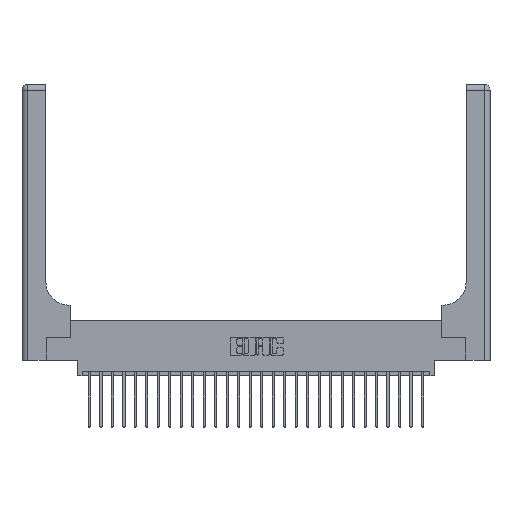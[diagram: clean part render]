
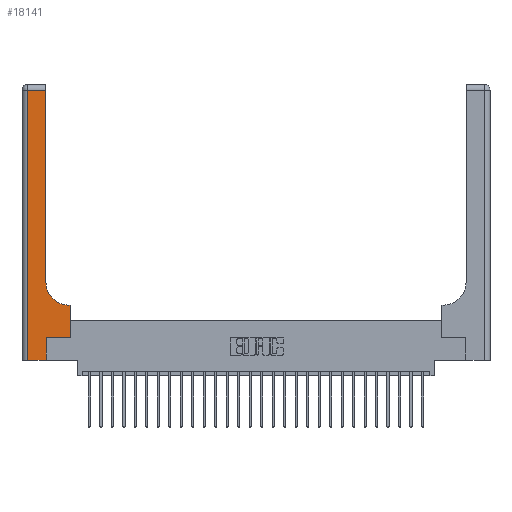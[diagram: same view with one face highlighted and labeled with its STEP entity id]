
A CAD part, top view. The second image highlights one B-rep face of the part: STEP entity #18141.
In plain terms, the highlighted planar face has unit normal (0, 0, 1).
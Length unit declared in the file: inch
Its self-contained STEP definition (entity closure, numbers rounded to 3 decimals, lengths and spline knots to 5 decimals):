
#2 = DIRECTION ( 'NONE',  ( 1., 0., 0. ) ) ;
#384 = DIRECTION ( 'NONE',  ( 0., 1., 0. ) ) ;
#414 = EDGE_CURVE ( 'NONE', #9148, #3747, #14140, .T. ) ;
#437 = CARTESIAN_POINT ( 'NONE',  ( 0.06, 3., 0.37 ) ) ;
#682 = CARTESIAN_POINT ( 'NONE',  ( 0.06, 0., 0.37 ) ) ;
#783 = CARTESIAN_POINT ( 'NONE',  ( 0.528, 0.6, 0.37 ) ) ;
#811 = DIRECTION ( 'NONE',  ( 1., 0., 0. ) ) ;
#1477 = LINE ( 'NONE', #24957, #22028 ) ;
#1727 = LINE ( 'NONE', #9113, #22916 ) ;
#2318 = DIRECTION ( 'NONE',  ( 1., 0., 0. ) ) ;
#2711 = VERTEX_POINT ( 'NONE', #22517 ) ;
#2744 = LINE ( 'NONE', #437, #19110 ) ;
#2953 = VERTEX_POINT ( 'NONE', #783 ) ;
#3747 = VERTEX_POINT ( 'NONE', #23976 ) ;
#4398 = CIRCLE ( 'NONE', #25524, 0.25 ) ;
#4482 = VECTOR ( 'NONE', #2318, 39.37008 ) ;
#4495 = LINE ( 'NONE', #6104, #14080 ) ;
#4912 = CARTESIAN_POINT ( 'NONE',  ( 0., 2.94, 0.37 ) ) ;
#4923 = FACE_OUTER_BOUND ( 'NONE', #15875, .T. ) ;
#5685 = VECTOR ( 'NONE', #19281, 39.37008 ) ;
#6093 = CARTESIAN_POINT ( 'NONE',  ( 0.51, 0.6, 0.37 ) ) ;
#6104 = CARTESIAN_POINT ( 'NONE',  ( 0.265, 0.25, 0.37 ) ) ;
#6271 = EDGE_CURVE ( 'NONE', #2711, #12326, #21415, .T. ) ;
#6777 = EDGE_CURVE ( 'NONE', #13794, #2711, #1477, .T. ) ;
#6854 = PLANE ( 'NONE',  #11545 ) ;
#7512 = ORIENTED_EDGE ( 'NONE', *, *, #14644, .T. ) ;
#7548 = CARTESIAN_POINT ( 'NONE',  ( 0.265, 0., 0.37 ) ) ;
#7654 = EDGE_CURVE ( 'NONE', #12326, #25879, #2744, .T. ) ;
#8391 = CARTESIAN_POINT ( 'NONE',  ( 0., 0., 0.37 ) ) ;
#8918 = DIRECTION ( 'NONE',  ( 0., 0., -1. ) ) ;
#9113 = CARTESIAN_POINT ( 'NONE',  ( 0.528, 0.25, 0.37 ) ) ;
#9148 = VERTEX_POINT ( 'NONE', #7548 ) ;
#10412 = EDGE_CURVE ( 'NONE', #22417, #13794, #4398, .T. ) ;
#10836 = ORIENTED_EDGE ( 'NONE', *, *, #17801, .T. ) ;
#11217 = DIRECTION ( 'NONE',  ( -1., 0., 0. ) ) ;
#11545 = AXIS2_PLACEMENT_3D ( 'NONE', #12942, #8918, #23276 ) ;
#11907 = CARTESIAN_POINT ( 'NONE',  ( 0.26, 0.85, 0.37 ) ) ;
#12326 = VERTEX_POINT ( 'NONE', #23500 ) ;
#12942 = CARTESIAN_POINT ( 'NONE',  ( 0., 3., 0.37 ) ) ;
#13046 = ORIENTED_EDGE ( 'NONE', *, *, #20359, .T. ) ;
#13093 = DIRECTION ( 'NONE',  ( 0., 1., 0. ) ) ;
#13095 = DIRECTION ( 'NONE',  ( 0., 0., -1. ) ) ;
#13794 = VERTEX_POINT ( 'NONE', #11907 ) ;
#14080 = VECTOR ( 'NONE', #2, 39.37008 ) ;
#14140 = LINE ( 'NONE', #21115, #19012 ) ;
#14644 = EDGE_CURVE ( 'NONE', #25879, #9148, #20851, .T. ) ;
#15049 = VECTOR ( 'NONE', #11217, 39.37008 ) ;
#15875 = EDGE_LOOP ( 'NONE', ( #20705, #19772, #24175, #7512, #19114, #13046, #10836, #22332, #19027 ) ) ;
#17546 = VERTEX_POINT ( 'NONE', #24544 ) ;
#17801 = EDGE_CURVE ( 'NONE', #17546, #2953, #1727, .T. ) ;
#18141 = ADVANCED_FACE ( 'NONE', ( #4923 ), #6854, .F. ) ;
#19012 = VECTOR ( 'NONE', #13093, 39.37008 ) ;
#19027 = ORIENTED_EDGE ( 'NONE', *, *, #10412, .T. ) ;
#19110 = VECTOR ( 'NONE', #20998, 39.37008 ) ;
#19114 = ORIENTED_EDGE ( 'NONE', *, *, #414, .T. ) ;
#19281 = DIRECTION ( 'NONE',  ( -1., 0., 0. ) ) ;
#19772 = ORIENTED_EDGE ( 'NONE', *, *, #6271, .T. ) ;
#20359 = EDGE_CURVE ( 'NONE', #3747, #17546, #4495, .T. ) ;
#20564 = LINE ( 'NONE', #21456, #15049 ) ;
#20705 = ORIENTED_EDGE ( 'NONE', *, *, #6777, .T. ) ;
#20851 = LINE ( 'NONE', #8391, #4482 ) ;
#20998 = DIRECTION ( 'NONE',  ( 0., -1., 0. ) ) ;
#21115 = CARTESIAN_POINT ( 'NONE',  ( 0.265, 0., 0.37 ) ) ;
#21415 = LINE ( 'NONE', #4912, #5685 ) ;
#21456 = CARTESIAN_POINT ( 'NONE',  ( 0.26, 0.6, 0.37 ) ) ;
#22028 = VECTOR ( 'NONE', #384, 39.37008 ) ;
#22332 = ORIENTED_EDGE ( 'NONE', *, *, #25313, .T. ) ;
#22417 = VERTEX_POINT ( 'NONE', #6093 ) ;
#22517 = CARTESIAN_POINT ( 'NONE',  ( 0.26, 2.94, 0.37 ) ) ;
#22916 = VECTOR ( 'NONE', #23469, 39.37008 ) ;
#23276 = DIRECTION ( 'NONE',  ( -1., 0., 0. ) ) ;
#23469 = DIRECTION ( 'NONE',  ( 0., 1., 0. ) ) ;
#23500 = CARTESIAN_POINT ( 'NONE',  ( 0.06, 2.94, 0.37 ) ) ;
#23976 = CARTESIAN_POINT ( 'NONE',  ( 0.265, 0.25, 0.37 ) ) ;
#24175 = ORIENTED_EDGE ( 'NONE', *, *, #7654, .T. ) ;
#24544 = CARTESIAN_POINT ( 'NONE',  ( 0.528, 0.25, 0.37 ) ) ;
#24957 = CARTESIAN_POINT ( 'NONE',  ( 0.26, 3., 0.37 ) ) ;
#25313 = EDGE_CURVE ( 'NONE', #2953, #22417, #20564, .T. ) ;
#25382 = CARTESIAN_POINT ( 'NONE',  ( 0.51, 0.85, 0.37 ) ) ;
#25524 = AXIS2_PLACEMENT_3D ( 'NONE', #25382, #13095, #811 ) ;
#25879 = VERTEX_POINT ( 'NONE', #682 ) ;
